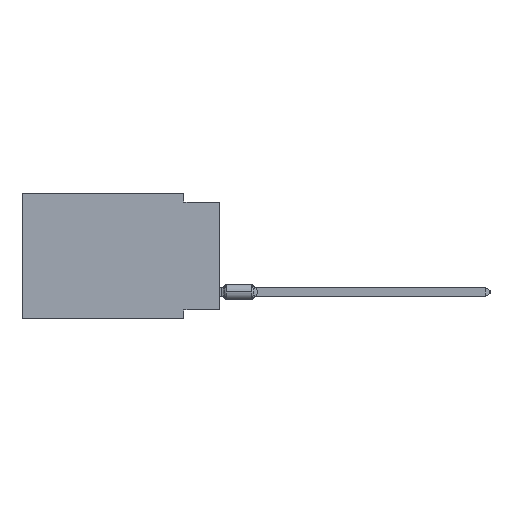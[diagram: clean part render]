
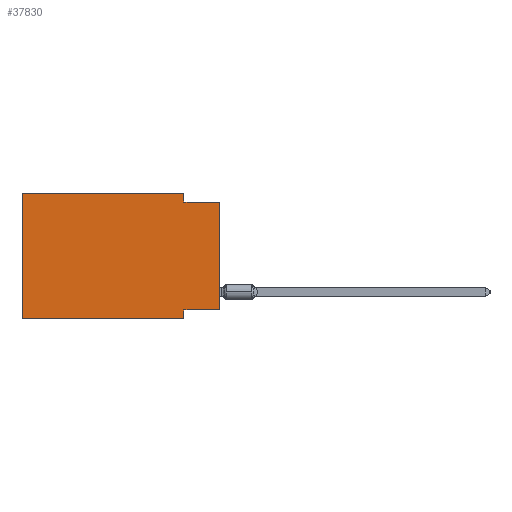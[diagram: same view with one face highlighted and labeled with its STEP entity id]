
A CAD part, left-side view. The second image highlights one B-rep face of the part: STEP entity #37830.
In plain terms, the highlighted planar face has unit normal (-1, 0, 0).
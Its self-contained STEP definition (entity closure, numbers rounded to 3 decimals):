
#1307 = LINE ( 'NONE', #34390, #20176 ) ;
#1537 = LINE ( 'NONE', #60072, #37375 ) ;
#3856 = CARTESIAN_POINT ( 'NONE',  ( 0., 2.54, -8.89 ) ) ;
#7842 = DIRECTION ( 'NONE',  ( 1., 0., 0. ) ) ;
#8050 = EDGE_CURVE ( 'NONE', #24043, #90909, #48865, .T. ) ;
#9410 = CARTESIAN_POINT ( 'NONE',  ( 0., 13.97, 0. ) ) ;
#10720 = CARTESIAN_POINT ( 'NONE',  ( 0., 13.97, -8.89 ) ) ;
#11339 = ORIENTED_EDGE ( 'NONE', *, *, #41998, .F. ) ;
#12106 = LINE ( 'NONE', #53823, #30203 ) ;
#12564 = DIRECTION ( 'NONE',  ( 0., -1., 0. ) ) ;
#13536 = ORIENTED_EDGE ( 'NONE', *, *, #8050, .F. ) ;
#14089 = CARTESIAN_POINT ( 'NONE',  ( 0., 0., -8.255 ) ) ;
#15120 = ORIENTED_EDGE ( 'NONE', *, *, #76050, .F. ) ;
#17125 = CARTESIAN_POINT ( 'NONE',  ( 0., 0., -8.255 ) ) ;
#17469 = ORIENTED_EDGE ( 'NONE', *, *, #105256, .F. ) ;
#19528 = VECTOR ( 'NONE', #77370, 1000. ) ;
#20176 = VECTOR ( 'NONE', #70638, 1000. ) ;
#21843 = LINE ( 'NONE', #32143, #50000 ) ;
#24043 = VERTEX_POINT ( 'NONE', #47053 ) ;
#24624 = EDGE_CURVE ( 'NONE', #90909, #66936, #21843, .T. ) ;
#25372 = ORIENTED_EDGE ( 'NONE', *, *, #39826, .F. ) ;
#25897 = VECTOR ( 'NONE', #12564, 1000. ) ;
#26003 = VERTEX_POINT ( 'NONE', #3856 ) ;
#26210 = PLANE ( 'NONE',  #49158 ) ;
#27367 = CARTESIAN_POINT ( 'NONE',  ( 0., 0., -0.635 ) ) ;
#27789 = LINE ( 'NONE', #86819, #25897 ) ;
#30203 = VECTOR ( 'NONE', #95010, 1000. ) ;
#31926 = ORIENTED_EDGE ( 'NONE', *, *, #32116, .T. ) ;
#32116 = EDGE_CURVE ( 'NONE', #51675, #26003, #12106, .T. ) ;
#32143 = CARTESIAN_POINT ( 'NONE',  ( 0., 2.54, 0. ) ) ;
#34390 = CARTESIAN_POINT ( 'NONE',  ( 0., 0., 0. ) ) ;
#37375 = VECTOR ( 'NONE', #100720, 1000. ) ;
#37702 = VECTOR ( 'NONE', #55279, 1000. ) ;
#37830 = ADVANCED_FACE ( 'NONE', ( #50062 ), #26210, .F. ) ;
#39826 = EDGE_CURVE ( 'NONE', #51675, #24043, #1537, .T. ) ;
#40961 = VERTEX_POINT ( 'NONE', #17125 ) ;
#41998 = EDGE_CURVE ( 'NONE', #40961, #105078, #71544, .T. ) ;
#47053 = CARTESIAN_POINT ( 'NONE',  ( 0., 13.97, 0. ) ) ;
#48865 = LINE ( 'NONE', #65668, #19528 ) ;
#49158 = AXIS2_PLACEMENT_3D ( 'NONE', #9410, #7842, #92311 ) ;
#50000 = VECTOR ( 'NONE', #81455, 1000. ) ;
#50062 = FACE_OUTER_BOUND ( 'NONE', #98408, .T. ) ;
#51675 = VERTEX_POINT ( 'NONE', #10720 ) ;
#53823 = CARTESIAN_POINT ( 'NONE',  ( 0., 13.97, -8.89 ) ) ;
#55279 = DIRECTION ( 'NONE',  ( 0., 1., 0. ) ) ;
#59064 = CARTESIAN_POINT ( 'NONE',  ( 0., 2.54, -8.255 ) ) ;
#59087 = ORIENTED_EDGE ( 'NONE', *, *, #24624, .F. ) ;
#60072 = CARTESIAN_POINT ( 'NONE',  ( 0., 13.97, 0. ) ) ;
#65668 = CARTESIAN_POINT ( 'NONE',  ( 0., 13.97, 0. ) ) ;
#66936 = VERTEX_POINT ( 'NONE', #85858 ) ;
#70638 = DIRECTION ( 'NONE',  ( 0., 0., 1. ) ) ;
#71544 = LINE ( 'NONE', #14089, #37702 ) ;
#76050 = EDGE_CURVE ( 'NONE', #66936, #97900, #27789, .T. ) ;
#76936 = LINE ( 'NONE', #101856, #81035 ) ;
#77370 = DIRECTION ( 'NONE',  ( 0., -1., 0. ) ) ;
#81035 = VECTOR ( 'NONE', #84002, 1000. ) ;
#81455 = DIRECTION ( 'NONE',  ( 0., 0., -1. ) ) ;
#84002 = DIRECTION ( 'NONE',  ( 0., 0., -1. ) ) ;
#85858 = CARTESIAN_POINT ( 'NONE',  ( 0., 2.54, -0.635 ) ) ;
#85957 = ORIENTED_EDGE ( 'NONE', *, *, #103584, .T. ) ;
#86819 = CARTESIAN_POINT ( 'NONE',  ( 0., 0., -0.635 ) ) ;
#90909 = VERTEX_POINT ( 'NONE', #97281 ) ;
#92311 = DIRECTION ( 'NONE',  ( 0., 0., -1. ) ) ;
#95010 = DIRECTION ( 'NONE',  ( 0., -1., 0. ) ) ;
#97281 = CARTESIAN_POINT ( 'NONE',  ( 0., 2.54, 0. ) ) ;
#97900 = VERTEX_POINT ( 'NONE', #27367 ) ;
#98408 = EDGE_LOOP ( 'NONE', ( #85957, #15120, #59087, #13536, #25372, #31926, #17469, #11339 ) ) ;
#100720 = DIRECTION ( 'NONE',  ( 0., 0., 1. ) ) ;
#101856 = CARTESIAN_POINT ( 'NONE',  ( 0., 2.54, -8.89 ) ) ;
#103584 = EDGE_CURVE ( 'NONE', #40961, #97900, #1307, .T. ) ;
#105078 = VERTEX_POINT ( 'NONE', #59064 ) ;
#105256 = EDGE_CURVE ( 'NONE', #105078, #26003, #76936, .T. ) ;
